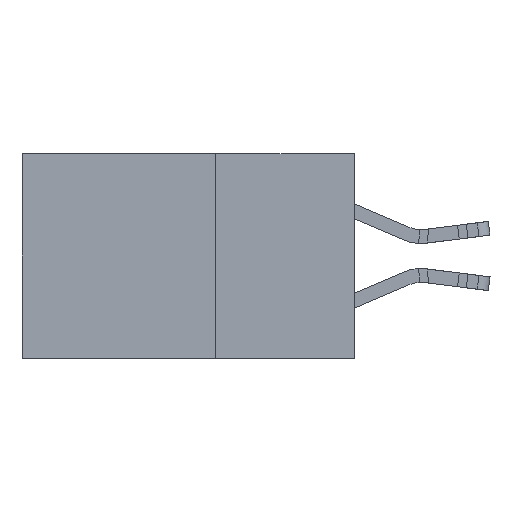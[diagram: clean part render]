
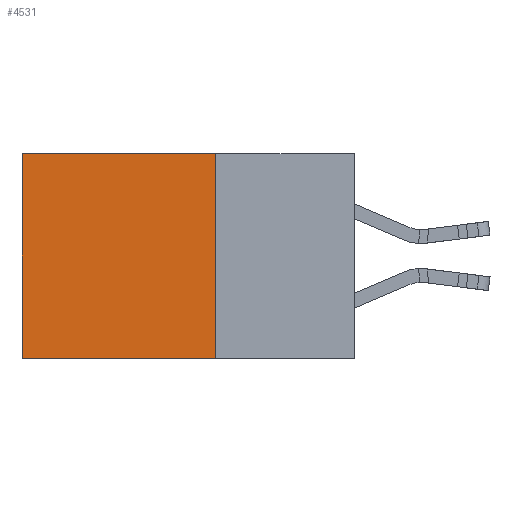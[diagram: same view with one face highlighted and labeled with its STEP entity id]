
A CAD part, left-side view. The second image highlights one B-rep face of the part: STEP entity #4531.
In plain terms, the highlighted planar face has unit normal (-1, 0, 0).
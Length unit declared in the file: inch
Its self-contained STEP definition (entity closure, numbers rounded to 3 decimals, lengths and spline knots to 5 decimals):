
#31 = CARTESIAN_POINT ( 'NONE',  ( 0.298, 0.25, -0.37 ) ) ;
#2264 = ORIENTED_EDGE ( 'NONE', *, *, #9322, .T. ) ;
#2644 = ORIENTED_EDGE ( 'NONE', *, *, #27040, .F. ) ;
#3449 = FACE_OUTER_BOUND ( 'NONE', #22752, .T. ) ;
#3922 = DIRECTION ( 'NONE',  ( 1., 0., 0. ) ) ;
#4531 = ADVANCED_FACE ( 'NONE', ( #3449 ), #25772, .F. ) ;
#4675 = VECTOR ( 'NONE', #6635, 39.37008 ) ;
#5000 = VERTEX_POINT ( 'NONE', #5756 ) ;
#5636 = VECTOR ( 'NONE', #9442, 39.37008 ) ;
#5673 = LINE ( 'NONE', #27103, #26670 ) ;
#5756 = CARTESIAN_POINT ( 'NONE',  ( 0.298, 0.6, 0. ) ) ;
#6635 = DIRECTION ( 'NONE',  ( 0., 0., -1. ) ) ;
#6693 = LINE ( 'NONE', #17040, #12293 ) ;
#9273 = VERTEX_POINT ( 'NONE', #31 ) ;
#9322 = EDGE_CURVE ( 'NONE', #21900, #5000, #6693, .T. ) ;
#9442 = DIRECTION ( 'NONE',  ( 0., 0., -1. ) ) ;
#9918 = AXIS2_PLACEMENT_3D ( 'NONE', #10992, #3922, #16013 ) ;
#10992 = CARTESIAN_POINT ( 'NONE',  ( 0.298, 0.25, 0. ) ) ;
#12293 = VECTOR ( 'NONE', #17134, 39.37008 ) ;
#14552 = CARTESIAN_POINT ( 'NONE',  ( 0.298, 0.6, -0.37 ) ) ;
#14706 = DIRECTION ( 'NONE',  ( 0., 1., 0. ) ) ;
#15611 = CARTESIAN_POINT ( 'NONE',  ( 0.298, 0.25, 0. ) ) ;
#16013 = DIRECTION ( 'NONE',  ( 0., 0., -1. ) ) ;
#17040 = CARTESIAN_POINT ( 'NONE',  ( 0.298, 0.25, 0. ) ) ;
#17134 = DIRECTION ( 'NONE',  ( 0., 1., 0. ) ) ;
#18275 = CARTESIAN_POINT ( 'NONE',  ( 0.298, 0.6, 0. ) ) ;
#18556 = EDGE_CURVE ( 'NONE', #21900, #9273, #29625, .T. ) ;
#18664 = VERTEX_POINT ( 'NONE', #14552 ) ;
#21392 = CARTESIAN_POINT ( 'NONE',  ( 0.298, 0.25, 0. ) ) ;
#21900 = VERTEX_POINT ( 'NONE', #15611 ) ;
#22752 = EDGE_LOOP ( 'NONE', ( #30615, #2644, #28872, #2264 ) ) ;
#25772 = PLANE ( 'NONE',  #9918 ) ;
#26670 = VECTOR ( 'NONE', #14706, 39.37008 ) ;
#27040 = EDGE_CURVE ( 'NONE', #9273, #18664, #5673, .T. ) ;
#27103 = CARTESIAN_POINT ( 'NONE',  ( 0.298, 0.25, -0.37 ) ) ;
#28872 = ORIENTED_EDGE ( 'NONE', *, *, #18556, .F. ) ;
#29625 = LINE ( 'NONE', #21392, #5636 ) ;
#29750 = LINE ( 'NONE', #18275, #4675 ) ;
#30615 = ORIENTED_EDGE ( 'NONE', *, *, #30962, .T. ) ;
#30962 = EDGE_CURVE ( 'NONE', #5000, #18664, #29750, .T. ) ;
